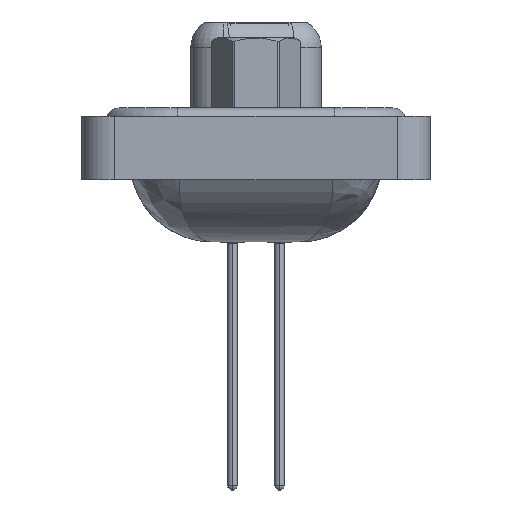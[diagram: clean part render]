
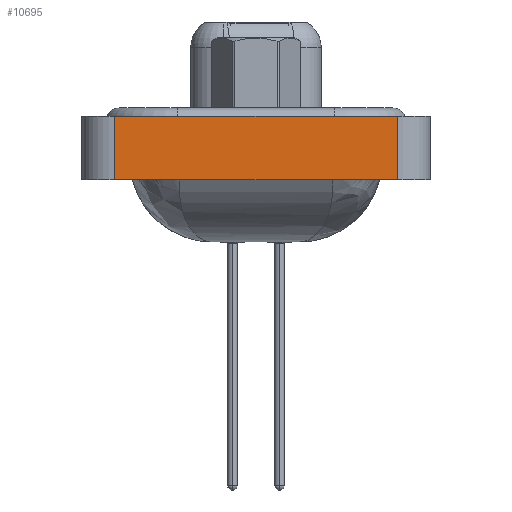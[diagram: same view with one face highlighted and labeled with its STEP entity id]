
A CAD part, left-side view. The second image highlights one B-rep face of the part: STEP entity #10695.
In plain terms, the highlighted planar face has unit normal (-1, 0, 0).
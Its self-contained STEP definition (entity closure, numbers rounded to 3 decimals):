
#481 = ORIENTED_EDGE ( 'NONE', *, *, #10784, .T. ) ;
#1645 = CARTESIAN_POINT ( 'NONE',  ( -7.225, -8.55, 0.5 ) ) ;
#2751 = DIRECTION ( 'NONE',  ( 0., 0., 1. ) ) ;
#3565 = ORIENTED_EDGE ( 'NONE', *, *, #3658, .T. ) ;
#3658 = EDGE_CURVE ( 'NONE', #12285, #19762, #19835, .T. ) ;
#4817 = DIRECTION ( 'NONE',  ( 0., 0., 1. ) ) ;
#5601 = AXIS2_PLACEMENT_3D ( 'NONE', #13346, #15826, #4817 ) ;
#5773 = VERTEX_POINT ( 'NONE', #27206 ) ;
#6099 = VERTEX_POINT ( 'NONE', #1645 ) ;
#10695 = ADVANCED_FACE ( 'NONE', ( #28907 ), #20071, .T. ) ;
#10784 = EDGE_CURVE ( 'NONE', #19762, #6099, #25349, .T. ) ;
#11834 = EDGE_CURVE ( 'NONE', #12285, #5773, #21253, .T. ) ;
#12285 = VERTEX_POINT ( 'NONE', #16267 ) ;
#13066 = VECTOR ( 'NONE', #28232, 1000. ) ;
#13346 = CARTESIAN_POINT ( 'NONE',  ( -7.225, -8.55, -3.35 ) ) ;
#13938 = CARTESIAN_POINT ( 'NONE',  ( -7.225, -8.55, -3.35 ) ) ;
#15028 = CARTESIAN_POINT ( 'NONE',  ( -7.225, -8.55, -3.35 ) ) ;
#15826 = DIRECTION ( 'NONE',  ( -1., 0., 0. ) ) ;
#16267 = CARTESIAN_POINT ( 'NONE',  ( -7.225, 8.55, -3.35 ) ) ;
#16317 = VECTOR ( 'NONE', #19525, 1000. ) ;
#16829 = VECTOR ( 'NONE', #2751, 1000. ) ;
#17191 = LINE ( 'NONE', #26272, #16317 ) ;
#17816 = ORIENTED_EDGE ( 'NONE', *, *, #27191, .F. ) ;
#18455 = EDGE_LOOP ( 'NONE', ( #481, #17816, #27167, #3565 ) ) ;
#19344 = CARTESIAN_POINT ( 'NONE',  ( -7.225, -8.55, -3.35 ) ) ;
#19525 = DIRECTION ( 'NONE',  ( 0., -1., 0. ) ) ;
#19762 = VERTEX_POINT ( 'NONE', #19344 ) ;
#19835 = LINE ( 'NONE', #15028, #13066 ) ;
#20071 = PLANE ( 'NONE',  #5601 ) ;
#20972 = CARTESIAN_POINT ( 'NONE',  ( -7.225, 8.55, -3.35 ) ) ;
#21253 = LINE ( 'NONE', #20972, #27654 ) ;
#25256 = DIRECTION ( 'NONE',  ( 0., 0., 1. ) ) ;
#25349 = LINE ( 'NONE', #13938, #16829 ) ;
#26272 = CARTESIAN_POINT ( 'NONE',  ( -7.225, -8.55, 0.5 ) ) ;
#27167 = ORIENTED_EDGE ( 'NONE', *, *, #11834, .F. ) ;
#27191 = EDGE_CURVE ( 'NONE', #5773, #6099, #17191, .T. ) ;
#27206 = CARTESIAN_POINT ( 'NONE',  ( -7.225, 8.55, 0.5 ) ) ;
#27654 = VECTOR ( 'NONE', #25256, 1000. ) ;
#28232 = DIRECTION ( 'NONE',  ( 0., -1., 0. ) ) ;
#28907 = FACE_OUTER_BOUND ( 'NONE', #18455, .T. ) ;
